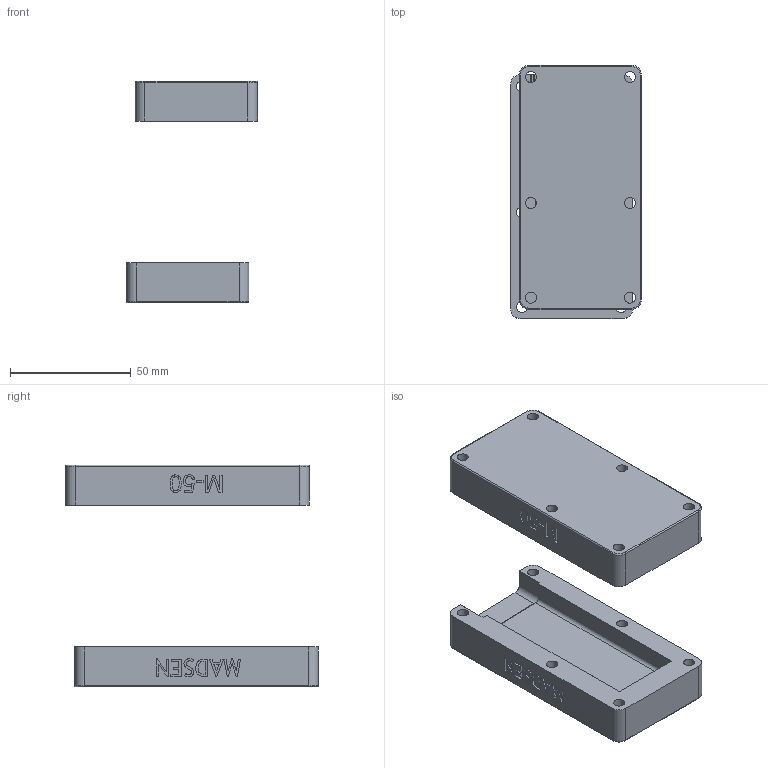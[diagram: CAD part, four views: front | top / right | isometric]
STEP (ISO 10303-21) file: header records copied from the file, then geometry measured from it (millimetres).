
FILE_DESCRIPTION(/* description */ (''),/* implementation_level */ '2;1');
FILE_NAME(/* name */ 'Madsen long magazine extension v9.step',/* time_stamp */ '2018-09-18T20:24:55-05:00',/* author */ ('greg.bestland'),/* organization */ (''),/* preprocessor_version */ 'ST-DEVELOPER v17.2',/* originating_system */ 'Autodesk Translation Framework v7.6.0.251',/* authorisation */ '');
FILE_SCHEMA (('AUTOMOTIVE_DESIGN { 1 0 10303 214 3 1 1 }'));
Length unit declared in the file: millimetre
Products named in the file (1): Madsen magazine extension
Bounding box: 54.28 x 104.74 x 91.75 mm (x, y, z)
Volume: 110770.7 mm3; surface area: 36854 mm2
Topology: 2 solids, 2 shells, 514 faces, 1408 edges, 931 vertices
Faces by surface type: plane 268, bspline 202, cylinder 36, torus 8
Full cylindrical faces by diameter (mm): 4.6 x12
Entity records: 18088 total; most frequent: CARTESIAN_POINT 6288, ORIENTED_EDGE 2816, DIRECTION 1710, EDGE_CURVE 1408, VERTEX_POINT 931, LINE 924, VECTOR 924, EDGE_LOOP 571
